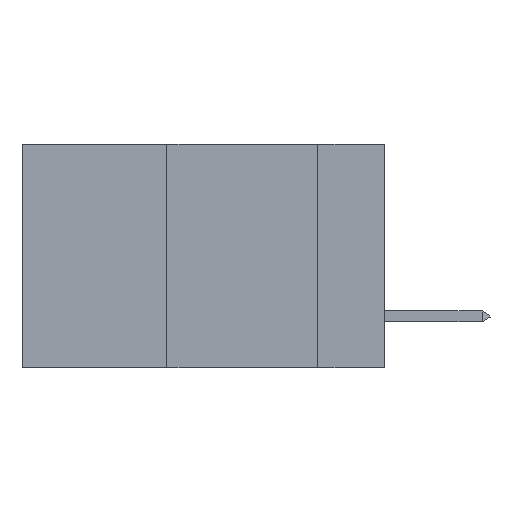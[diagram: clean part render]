
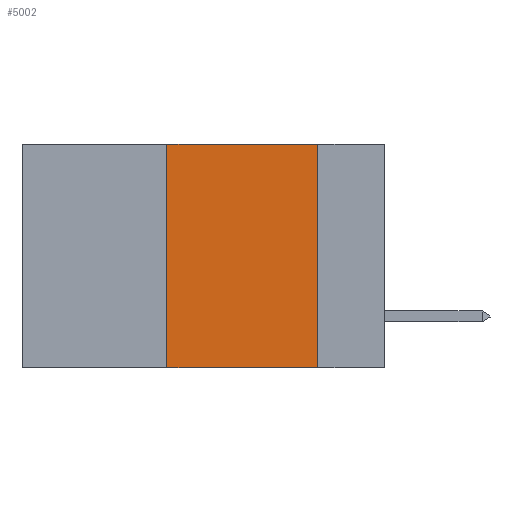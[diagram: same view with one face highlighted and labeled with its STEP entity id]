
A CAD part, left-side view. The second image highlights one B-rep face of the part: STEP entity #5002.
In plain terms, the highlighted planar face has unit normal (-1, 0, 0).
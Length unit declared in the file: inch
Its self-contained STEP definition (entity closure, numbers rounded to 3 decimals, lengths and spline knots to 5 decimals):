
#2 = CARTESIAN_POINT ( 'NONE',  ( 0., 0.36, 0. ) ) ;
#31 = EDGE_LOOP ( 'NONE', ( #10683, #3354, #5575, #18899 ) ) ;
#146 = DIRECTION ( 'NONE',  ( 1., 0., 0. ) ) ;
#1382 = VECTOR ( 'NONE', #2869, 39.37008 ) ;
#2869 = DIRECTION ( 'NONE',  ( 0., -1., 0. ) ) ;
#3354 = ORIENTED_EDGE ( 'NONE', *, *, #4074, .F. ) ;
#3660 = CARTESIAN_POINT ( 'NONE',  ( 0., 0.36, 0. ) ) ;
#4074 = EDGE_CURVE ( 'NONE', #20256, #22508, #18390, .T. ) ;
#4570 = FACE_OUTER_BOUND ( 'NONE', #31, .T. ) ;
#5002 = ADVANCED_FACE ( 'NONE', ( #4570 ), #12309, .F. ) ;
#5575 = ORIENTED_EDGE ( 'NONE', *, *, #11491, .F. ) ;
#6077 = EDGE_CURVE ( 'NONE', #19306, #9741, #18145, .T. ) ;
#6450 = CARTESIAN_POINT ( 'NONE',  ( 0., 0.11, 0. ) ) ;
#8301 = CARTESIAN_POINT ( 'NONE',  ( 0., 0.6, 0. ) ) ;
#8978 = CARTESIAN_POINT ( 'NONE',  ( 0., 0.6, -0.37 ) ) ;
#9741 = VERTEX_POINT ( 'NONE', #10580 ) ;
#10580 = CARTESIAN_POINT ( 'NONE',  ( 0., 0.11, -0.37 ) ) ;
#10683 = ORIENTED_EDGE ( 'NONE', *, *, #25839, .F. ) ;
#11491 = EDGE_CURVE ( 'NONE', #19306, #20256, #18251, .T. ) ;
#12309 = PLANE ( 'NONE',  #12608 ) ;
#12608 = AXIS2_PLACEMENT_3D ( 'NONE', #8301, #146, #18218 ) ;
#12894 = DIRECTION ( 'NONE',  ( 0., 0., -1. ) ) ;
#16104 = DIRECTION ( 'NONE',  ( 0., 0., 1. ) ) ;
#17876 = DIRECTION ( 'NONE',  ( 0., -1., 0. ) ) ;
#18145 = LINE ( 'NONE', #8978, #1382 ) ;
#18218 = DIRECTION ( 'NONE',  ( 0., 0., -1. ) ) ;
#18251 = LINE ( 'NONE', #2, #20432 ) ;
#18390 = LINE ( 'NONE', #23879, #22457 ) ;
#18899 = ORIENTED_EDGE ( 'NONE', *, *, #6077, .T. ) ;
#19306 = VERTEX_POINT ( 'NONE', #20442 ) ;
#19464 = VECTOR ( 'NONE', #12894, 39.37008 ) ;
#20256 = VERTEX_POINT ( 'NONE', #3660 ) ;
#20432 = VECTOR ( 'NONE', #16104, 39.37008 ) ;
#20442 = CARTESIAN_POINT ( 'NONE',  ( 0., 0.36, -0.37 ) ) ;
#22457 = VECTOR ( 'NONE', #17876, 39.37008 ) ;
#22508 = VERTEX_POINT ( 'NONE', #6450 ) ;
#22949 = CARTESIAN_POINT ( 'NONE',  ( 0., 0.11, 0. ) ) ;
#23879 = CARTESIAN_POINT ( 'NONE',  ( 0., 0.6, 0. ) ) ;
#25480 = LINE ( 'NONE', #22949, #19464 ) ;
#25839 = EDGE_CURVE ( 'NONE', #22508, #9741, #25480, .T. ) ;
